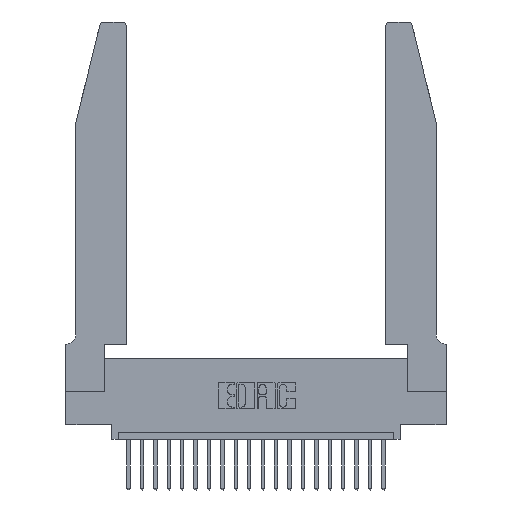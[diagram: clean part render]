
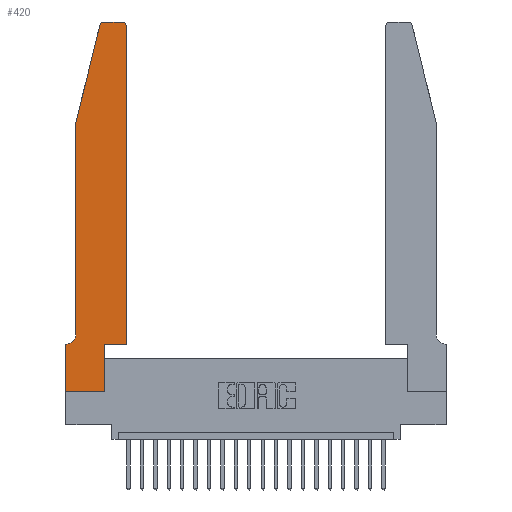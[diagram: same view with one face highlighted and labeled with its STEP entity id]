
A CAD part, top view. The second image highlights one B-rep face of the part: STEP entity #420.
In plain terms, the highlighted planar face has unit normal (0, 0, 1).
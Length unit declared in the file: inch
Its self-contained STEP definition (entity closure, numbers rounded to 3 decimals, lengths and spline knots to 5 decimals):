
#7 = ORIENTED_EDGE ( 'NONE', *, *, #2242, .T. ) ;
#280 = ORIENTED_EDGE ( 'NONE', *, *, #20294, .T. ) ;
#420 = ADVANCED_FACE ( 'NONE', ( #17977 ), #11799, .T. ) ;
#565 = CARTESIAN_POINT ( 'NONE',  ( 0.4505, 0.35, 0.37 ) ) ;
#797 = DIRECTION ( 'NONE',  ( 0., 0., -1. ) ) ;
#1025 = CARTESIAN_POINT ( 'NONE',  ( 0.4505, 0.35, 0.37 ) ) ;
#1216 = AXIS2_PLACEMENT_3D ( 'NONE', #18538, #797, #7888 ) ;
#1291 = CARTESIAN_POINT ( 'NONE',  ( 0.4205, 2.72, 0.37 ) ) ;
#1314 = VECTOR ( 'NONE', #15506, 39.37008 ) ;
#1365 = DIRECTION ( 'NONE',  ( 1., 0., 0. ) ) ;
#1867 = VERTEX_POINT ( 'NONE', #3275 ) ;
#2242 = EDGE_CURVE ( 'NONE', #16124, #14191, #18163, .T. ) ;
#2448 = CIRCLE ( 'NONE', #17394, 0.03 ) ;
#2491 = DIRECTION ( 'NONE',  ( 1., 0., 0. ) ) ;
#2799 = DIRECTION ( 'NONE',  ( 0., 1., 0. ) ) ;
#2896 = CARTESIAN_POINT ( 'NONE',  ( 0., 0.35, 0.37 ) ) ;
#2897 = ORIENTED_EDGE ( 'NONE', *, *, #12984, .T. ) ;
#2935 = CARTESIAN_POINT ( 'NONE',  ( 0.0755, 2., 0.37 ) ) ;
#3053 = CARTESIAN_POINT ( 'NONE',  ( 0.0755, 0.35, 0.37 ) ) ;
#3136 = CARTESIAN_POINT ( 'NONE',  ( 0., 0., 0.37 ) ) ;
#3275 = CARTESIAN_POINT ( 'NONE',  ( 0.2865, 0.35, 0.37 ) ) ;
#4121 = DIRECTION ( 'NONE',  ( -1., 0., 0. ) ) ;
#4284 = CARTESIAN_POINT ( 'NONE',  ( 0.4505, 2.72, 0.37 ) ) ;
#4586 = DIRECTION ( 'NONE',  ( -1., 0., 0. ) ) ;
#4623 = DIRECTION ( 'NONE',  ( 0., 1., 0. ) ) ;
#4755 = EDGE_CURVE ( 'NONE', #18673, #14758, #2448, .T. ) ;
#4771 = CARTESIAN_POINT ( 'NONE',  ( 0.0755, 2., 0.37 ) ) ;
#5397 = LINE ( 'NONE', #4771, #6768 ) ;
#5859 = EDGE_LOOP ( 'NONE', ( #12025, #14058, #18680, #13504, #15447, #280, #7, #2897, #18644, #7152, #8972, #10778 ) ) ;
#5974 = LINE ( 'NONE', #565, #14843 ) ;
#6099 = EDGE_CURVE ( 'NONE', #1867, #20525, #5974, .T. ) ;
#6159 = EDGE_CURVE ( 'NONE', #20525, #17353, #12072, .T. ) ;
#6490 = CARTESIAN_POINT ( 'NONE',  ( 0.2865, 0., 0.37 ) ) ;
#6768 = VECTOR ( 'NONE', #11607, 39.37008 ) ;
#6784 = LINE ( 'NONE', #22371, #20412 ) ;
#7152 = ORIENTED_EDGE ( 'NONE', *, *, #6099, .T. ) ;
#7185 = EDGE_CURVE ( 'NONE', #22437, #18673, #11211, .T. ) ;
#7888 = DIRECTION ( 'NONE',  ( -1., 0., 0. ) ) ;
#7953 = LINE ( 'NONE', #3136, #1314 ) ;
#7998 = CARTESIAN_POINT ( 'NONE',  ( 0.284, 2.75, 0.37 ) ) ;
#8122 = DIRECTION ( 'NONE',  ( 0., -1., 0. ) ) ;
#8173 = CARTESIAN_POINT ( 'NONE',  ( 0.284, 2.72, 0.37 ) ) ;
#8200 = CARTESIAN_POINT ( 'NONE',  ( 0., 0., 0.37 ) ) ;
#8249 = DIRECTION ( 'NONE',  ( 1., 0., 0. ) ) ;
#8972 = ORIENTED_EDGE ( 'NONE', *, *, #6159, .T. ) ;
#9495 = CARTESIAN_POINT ( 'NONE',  ( 0.0755, 2., 0.37 ) ) ;
#10778 = ORIENTED_EDGE ( 'NONE', *, *, #15867, .T. ) ;
#10912 = LINE ( 'NONE', #2935, #20595 ) ;
#10993 = VERTEX_POINT ( 'NONE', #16238 ) ;
#11211 = LINE ( 'NONE', #16581, #20893 ) ;
#11356 = LINE ( 'NONE', #3053, #11887 ) ;
#11532 = VECTOR ( 'NONE', #2799, 39.37008 ) ;
#11607 = DIRECTION ( 'NONE',  ( 0., -1., 0. ) ) ;
#11617 = DIRECTION ( 'NONE',  ( -0.239, -0.971, 0. ) ) ;
#11799 = PLANE ( 'NONE',  #16304 ) ;
#11887 = VECTOR ( 'NONE', #4586, 39.37008 ) ;
#12025 = ORIENTED_EDGE ( 'NONE', *, *, #7185, .T. ) ;
#12072 = LINE ( 'NONE', #1025, #11532 ) ;
#12617 = CARTESIAN_POINT ( 'NONE',  ( 0., 0.35, 0.37 ) ) ;
#12984 = EDGE_CURVE ( 'NONE', #14191, #17789, #7953, .T. ) ;
#13337 = AXIS2_PLACEMENT_3D ( 'NONE', #1291, #13737, #1365 ) ;
#13504 = ORIENTED_EDGE ( 'NONE', *, *, #14520, .T. ) ;
#13737 = DIRECTION ( 'NONE',  ( 0., 0., 1. ) ) ;
#14058 = ORIENTED_EDGE ( 'NONE', *, *, #4755, .T. ) ;
#14191 = VERTEX_POINT ( 'NONE', #19281 ) ;
#14520 = EDGE_CURVE ( 'NONE', #15776, #18946, #5397, .T. ) ;
#14560 = CARTESIAN_POINT ( 'NONE',  ( 0.4505, 0.35, 0.37 ) ) ;
#14758 = VERTEX_POINT ( 'NONE', #14865 ) ;
#14843 = VECTOR ( 'NONE', #2491, 39.37008 ) ;
#14865 = CARTESIAN_POINT ( 'NONE',  ( 0.25487, 2.72718, 0.37 ) ) ;
#15267 = DIRECTION ( 'NONE',  ( 1., 0., 0. ) ) ;
#15447 = ORIENTED_EDGE ( 'NONE', *, *, #18665, .T. ) ;
#15506 = DIRECTION ( 'NONE',  ( 1., 0., 0. ) ) ;
#15776 = VERTEX_POINT ( 'NONE', #9495 ) ;
#15867 = EDGE_CURVE ( 'NONE', #17353, #22437, #20773, .T. ) ;
#16124 = VERTEX_POINT ( 'NONE', #12617 ) ;
#16238 = CARTESIAN_POINT ( 'NONE',  ( 0.0055, 0.35, 0.37 ) ) ;
#16304 = AXIS2_PLACEMENT_3D ( 'NONE', #2896, #16826, #15267 ) ;
#16581 = CARTESIAN_POINT ( 'NONE',  ( 0.2605, 2.75, 0.37 ) ) ;
#16680 = CIRCLE ( 'NONE', #1216, 0.07 ) ;
#16826 = DIRECTION ( 'NONE',  ( 0., 0., 1. ) ) ;
#17245 = EDGE_CURVE ( 'NONE', #14758, #15776, #10912, .T. ) ;
#17353 = VERTEX_POINT ( 'NONE', #4284 ) ;
#17394 = AXIS2_PLACEMENT_3D ( 'NONE', #8173, #20584, #8249 ) ;
#17735 = CARTESIAN_POINT ( 'NONE',  ( 0.0755, 0.42, 0.37 ) ) ;
#17789 = VERTEX_POINT ( 'NONE', #6490 ) ;
#17977 = FACE_OUTER_BOUND ( 'NONE', #5859, .T. ) ;
#18163 = LINE ( 'NONE', #8200, #19547 ) ;
#18538 = CARTESIAN_POINT ( 'NONE',  ( 0.0055, 0.42, 0.37 ) ) ;
#18644 = ORIENTED_EDGE ( 'NONE', *, *, #22139, .T. ) ;
#18665 = EDGE_CURVE ( 'NONE', #18946, #10993, #16680, .T. ) ;
#18673 = VERTEX_POINT ( 'NONE', #7998 ) ;
#18680 = ORIENTED_EDGE ( 'NONE', *, *, #17245, .T. ) ;
#18946 = VERTEX_POINT ( 'NONE', #17735 ) ;
#19281 = CARTESIAN_POINT ( 'NONE',  ( 0., 0., 0.37 ) ) ;
#19547 = VECTOR ( 'NONE', #8122, 39.37008 ) ;
#20294 = EDGE_CURVE ( 'NONE', #10993, #16124, #11356, .T. ) ;
#20412 = VECTOR ( 'NONE', #4623, 39.37008 ) ;
#20525 = VERTEX_POINT ( 'NONE', #14560 ) ;
#20584 = DIRECTION ( 'NONE',  ( 0., 0., 1. ) ) ;
#20595 = VECTOR ( 'NONE', #11617, 39.37008 ) ;
#20773 = CIRCLE ( 'NONE', #13337, 0.03 ) ;
#20893 = VECTOR ( 'NONE', #4121, 39.37008 ) ;
#21358 = CARTESIAN_POINT ( 'NONE',  ( 0.4205, 2.75, 0.37 ) ) ;
#22139 = EDGE_CURVE ( 'NONE', #17789, #1867, #6784, .T. ) ;
#22371 = CARTESIAN_POINT ( 'NONE',  ( 0.2865, 0.35, 0.37 ) ) ;
#22437 = VERTEX_POINT ( 'NONE', #21358 ) ;
